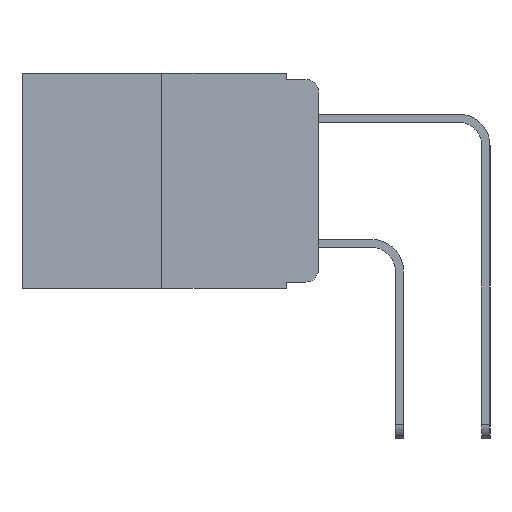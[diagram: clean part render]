
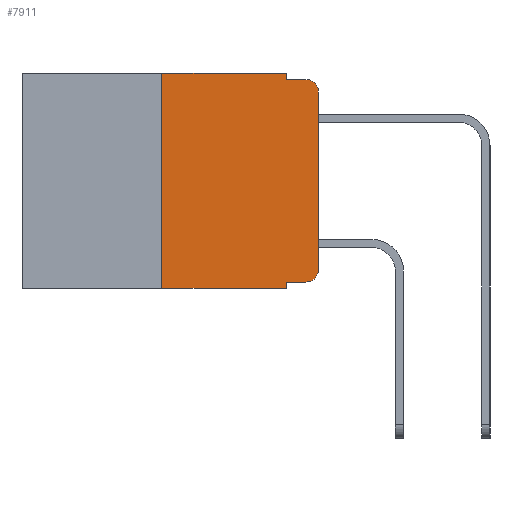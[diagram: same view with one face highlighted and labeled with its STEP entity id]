
A CAD part, left-side view. The second image highlights one B-rep face of the part: STEP entity #7911.
In plain terms, the highlighted planar face has unit normal (-1, 0, 0).
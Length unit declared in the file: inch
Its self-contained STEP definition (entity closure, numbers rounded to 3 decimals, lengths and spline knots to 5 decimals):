
#47 = CARTESIAN_POINT ( 'NONE',  ( 0., 0.25, 0. ) ) ;
#104 = CARTESIAN_POINT ( 'NONE',  ( 0., 0.02, -0.01 ) ) ;
#270 = DIRECTION ( 'NONE',  ( 0., 0., -1. ) ) ;
#321 = LINE ( 'NONE', #6497, #6520 ) ;
#387 = EDGE_CURVE ( 'NONE', #3466, #13747, #3057, .T. ) ;
#490 = CARTESIAN_POINT ( 'NONE',  ( 0., 0.02, -0.313 ) ) ;
#767 = CARTESIAN_POINT ( 'NONE',  ( 0., 0.051, -0.333 ) ) ;
#825 = VERTEX_POINT ( 'NONE', #12687 ) ;
#924 = EDGE_LOOP ( 'NONE', ( #10469, #10588, #10900, #11064, #9650, #9625, #9350, #9309, #9001, #8755 ) ) ;
#1018 = DIRECTION ( 'NONE',  ( 0., 0., 1. ) ) ;
#1388 = LINE ( 'NONE', #3729, #7141 ) ;
#1813 = DIRECTION ( 'NONE',  ( 0., 0., -1. ) ) ;
#1845 = CARTESIAN_POINT ( 'NONE',  ( 0., 0.473, -0.343 ) ) ;
#1988 = VERTEX_POINT ( 'NONE', #104 ) ;
#3057 = LINE ( 'NONE', #11514, #9057 ) ;
#3229 = DIRECTION ( 'NONE',  ( 0., 0., -1. ) ) ;
#3326 = EDGE_CURVE ( 'NONE', #5633, #1988, #5551, .T. ) ;
#3380 = DIRECTION ( 'NONE',  ( -1., 0., 0. ) ) ;
#3466 = VERTEX_POINT ( 'NONE', #767 ) ;
#3729 = CARTESIAN_POINT ( 'NONE',  ( 0., 0.473, 0. ) ) ;
#3804 = CARTESIAN_POINT ( 'NONE',  ( 0., 0.051, -0.343 ) ) ;
#3883 = CARTESIAN_POINT ( 'NONE',  ( 0., 0.473, 0. ) ) ;
#4152 = CARTESIAN_POINT ( 'NONE',  ( 0., 0.051, -0.01 ) ) ;
#4544 = AXIS2_PLACEMENT_3D ( 'NONE', #490, #9061, #1813 ) ;
#4919 = VERTEX_POINT ( 'NONE', #9320 ) ;
#5132 = EDGE_CURVE ( 'NONE', #15292, #10266, #5863, .T. ) ;
#5179 = VECTOR ( 'NONE', #9590, 39.37008 ) ;
#5425 = VECTOR ( 'NONE', #270, 39.37008 ) ;
#5551 = LINE ( 'NONE', #10362, #5179 ) ;
#5594 = AXIS2_PLACEMENT_3D ( 'NONE', #3883, #14474, #7516 ) ;
#5611 = FACE_OUTER_BOUND ( 'NONE', #924, .T. ) ;
#5633 = VERTEX_POINT ( 'NONE', #4152 ) ;
#5863 = LINE ( 'NONE', #1845, #9398 ) ;
#5932 = CARTESIAN_POINT ( 'NONE',  ( 0., 0.02, -0.333 ) ) ;
#6121 = EDGE_CURVE ( 'NONE', #9052, #13824, #1388, .T. ) ;
#6497 = CARTESIAN_POINT ( 'NONE',  ( 0., 0.25, 0. ) ) ;
#6520 = VECTOR ( 'NONE', #7733, 39.37008 ) ;
#7141 = VECTOR ( 'NONE', #9661, 39.37008 ) ;
#7439 = EDGE_CURVE ( 'NONE', #825, #1988, #11156, .T. ) ;
#7465 = PLANE ( 'NONE',  #5594 ) ;
#7516 = DIRECTION ( 'NONE',  ( 0., 0., -1. ) ) ;
#7733 = DIRECTION ( 'NONE',  ( 0., 0., 1. ) ) ;
#7746 = EDGE_CURVE ( 'NONE', #4919, #825, #14044, .T. ) ;
#7911 = ADVANCED_FACE ( 'NONE', ( #5611 ), #7465, .F. ) ;
#8015 = EDGE_CURVE ( 'NONE', #15292, #9052, #321, .T. ) ;
#8755 = ORIENTED_EDGE ( 'NONE', *, *, #12231, .T. ) ;
#8964 = LINE ( 'NONE', #11467, #14744 ) ;
#9001 = ORIENTED_EDGE ( 'NONE', *, *, #387, .T. ) ;
#9052 = VERTEX_POINT ( 'NONE', #47 ) ;
#9057 = VECTOR ( 'NONE', #9187, 39.37008 ) ;
#9061 = DIRECTION ( 'NONE',  ( -1., 0., 0. ) ) ;
#9187 = DIRECTION ( 'NONE',  ( 0., -1., 0. ) ) ;
#9301 = EDGE_CURVE ( 'NONE', #13824, #5633, #8964, .T. ) ;
#9309 = ORIENTED_EDGE ( 'NONE', *, *, #9767, .F. ) ;
#9320 = CARTESIAN_POINT ( 'NONE',  ( 0., 0., -0.313 ) ) ;
#9350 = ORIENTED_EDGE ( 'NONE', *, *, #5132, .T. ) ;
#9398 = VECTOR ( 'NONE', #12263, 39.37008 ) ;
#9590 = DIRECTION ( 'NONE',  ( 0., -1., 0. ) ) ;
#9625 = ORIENTED_EDGE ( 'NONE', *, *, #8015, .F. ) ;
#9650 = ORIENTED_EDGE ( 'NONE', *, *, #6121, .F. ) ;
#9661 = DIRECTION ( 'NONE',  ( 0., -1., 0. ) ) ;
#9767 = EDGE_CURVE ( 'NONE', #3466, #10266, #11673, .T. ) ;
#9839 = CARTESIAN_POINT ( 'NONE',  ( 0., 0.02, -0.03 ) ) ;
#10030 = CARTESIAN_POINT ( 'NONE',  ( 0., 0.051, 0. ) ) ;
#10138 = AXIS2_PLACEMENT_3D ( 'NONE', #9839, #3380, #3229 ) ;
#10157 = CIRCLE ( 'NONE', #4544, 0.02 ) ;
#10235 = VECTOR ( 'NONE', #1018, 39.37008 ) ;
#10266 = VERTEX_POINT ( 'NONE', #3804 ) ;
#10362 = CARTESIAN_POINT ( 'NONE',  ( 0., 0.051, -0.01 ) ) ;
#10469 = ORIENTED_EDGE ( 'NONE', *, *, #7746, .T. ) ;
#10588 = ORIENTED_EDGE ( 'NONE', *, *, #7439, .T. ) ;
#10900 = ORIENTED_EDGE ( 'NONE', *, *, #3326, .F. ) ;
#11064 = ORIENTED_EDGE ( 'NONE', *, *, #9301, .F. ) ;
#11156 = CIRCLE ( 'NONE', #10138, 0.02 ) ;
#11467 = CARTESIAN_POINT ( 'NONE',  ( 0., 0.051, 0. ) ) ;
#11514 = CARTESIAN_POINT ( 'NONE',  ( 0., 0.051, -0.333 ) ) ;
#11673 = LINE ( 'NONE', #10030, #5425 ) ;
#12231 = EDGE_CURVE ( 'NONE', #13747, #4919, #10157, .T. ) ;
#12263 = DIRECTION ( 'NONE',  ( 0., -1., 0. ) ) ;
#12574 = CARTESIAN_POINT ( 'NONE',  ( 0., 0.25, -0.343 ) ) ;
#12687 = CARTESIAN_POINT ( 'NONE',  ( 0., 0., -0.03 ) ) ;
#13747 = VERTEX_POINT ( 'NONE', #5932 ) ;
#13804 = DIRECTION ( 'NONE',  ( 0., 0., -1. ) ) ;
#13824 = VERTEX_POINT ( 'NONE', #15386 ) ;
#14044 = LINE ( 'NONE', #14133, #10235 ) ;
#14133 = CARTESIAN_POINT ( 'NONE',  ( 0., 0., 0. ) ) ;
#14474 = DIRECTION ( 'NONE',  ( 1., 0., 0. ) ) ;
#14744 = VECTOR ( 'NONE', #13804, 39.37008 ) ;
#15292 = VERTEX_POINT ( 'NONE', #12574 ) ;
#15386 = CARTESIAN_POINT ( 'NONE',  ( 0., 0.051, 0. ) ) ;
